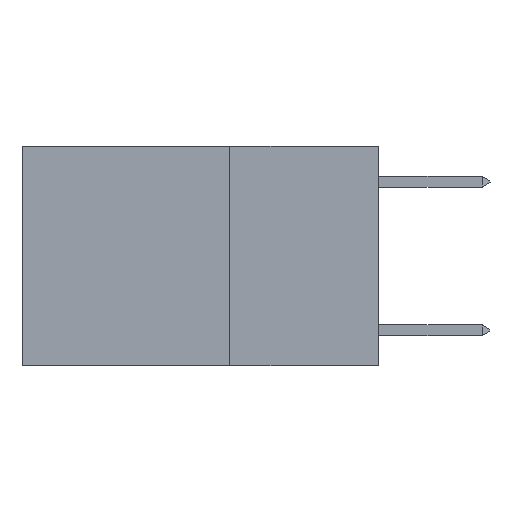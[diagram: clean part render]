
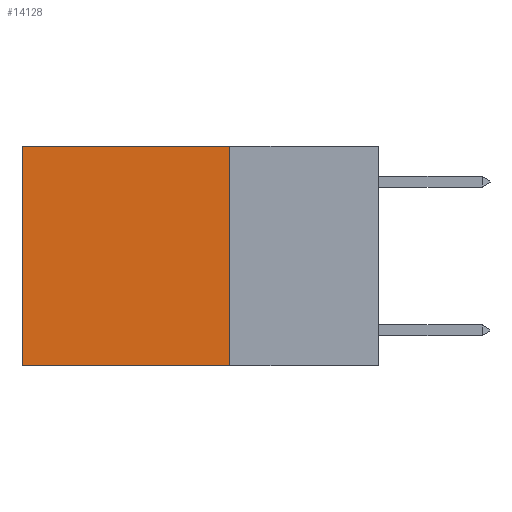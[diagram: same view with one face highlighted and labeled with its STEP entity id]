
A CAD part, left-side view. The second image highlights one B-rep face of the part: STEP entity #14128.
In plain terms, the highlighted planar face has unit normal (-1, 0, 0).
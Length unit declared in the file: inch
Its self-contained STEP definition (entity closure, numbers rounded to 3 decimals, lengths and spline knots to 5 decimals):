
#1373 = EDGE_CURVE ( 'NONE', #7896, #14406, #5699, .T. ) ;
#2200 = ORIENTED_EDGE ( 'NONE', *, *, #1373, .T. ) ;
#2500 = PLANE ( 'NONE',  #10295 ) ;
#2777 = EDGE_CURVE ( 'NONE', #14406, #12462, #14905, .T. ) ;
#3113 = LINE ( 'NONE', #14307, #6785 ) ;
#3574 = ORIENTED_EDGE ( 'NONE', *, *, #3704, .F. ) ;
#3704 = EDGE_CURVE ( 'NONE', #7896, #12253, #3113, .T. ) ;
#3740 = DIRECTION ( 'NONE',  ( 1., 0., 0. ) ) ;
#3807 = CARTESIAN_POINT ( 'NONE',  ( 0.2625, 0.25, 0. ) ) ;
#4279 = CARTESIAN_POINT ( 'NONE',  ( 0.2625, 0.6, 0. ) ) ;
#5164 = ORIENTED_EDGE ( 'NONE', *, *, #13948, .F. ) ;
#5699 = LINE ( 'NONE', #7059, #8932 ) ;
#5845 = VECTOR ( 'NONE', #6746, 39.37008 ) ;
#6357 = CARTESIAN_POINT ( 'NONE',  ( 0.2625, 0.25, -0.37 ) ) ;
#6698 = CARTESIAN_POINT ( 'NONE',  ( 0.2625, 0.6, 0. ) ) ;
#6746 = DIRECTION ( 'NONE',  ( 0., 0., -1. ) ) ;
#6785 = VECTOR ( 'NONE', #7250, 39.37008 ) ;
#7022 = VECTOR ( 'NONE', #9453, 39.37008 ) ;
#7059 = CARTESIAN_POINT ( 'NONE',  ( 0.2625, 0.25, 0. ) ) ;
#7250 = DIRECTION ( 'NONE',  ( 0., 0., -1. ) ) ;
#7896 = VERTEX_POINT ( 'NONE', #3807 ) ;
#7949 = FACE_OUTER_BOUND ( 'NONE', #11329, .T. ) ;
#8238 = CARTESIAN_POINT ( 'NONE',  ( 0.2625, 0.25, -0.37 ) ) ;
#8932 = VECTOR ( 'NONE', #15290, 39.37008 ) ;
#9453 = DIRECTION ( 'NONE',  ( 0., 1., 0. ) ) ;
#10246 = CARTESIAN_POINT ( 'NONE',  ( 0.2625, 0.6, -0.37 ) ) ;
#10295 = AXIS2_PLACEMENT_3D ( 'NONE', #14440, #3740, #12163 ) ;
#11329 = EDGE_LOOP ( 'NONE', ( #15172, #5164, #3574, #2200 ) ) ;
#12163 = DIRECTION ( 'NONE',  ( 0., 0., -1. ) ) ;
#12253 = VERTEX_POINT ( 'NONE', #6357 ) ;
#12462 = VERTEX_POINT ( 'NONE', #10246 ) ;
#13310 = LINE ( 'NONE', #8238, #7022 ) ;
#13948 = EDGE_CURVE ( 'NONE', #12253, #12462, #13310, .T. ) ;
#14128 = ADVANCED_FACE ( 'NONE', ( #7949 ), #2500, .F. ) ;
#14307 = CARTESIAN_POINT ( 'NONE',  ( 0.2625, 0.25, 0. ) ) ;
#14406 = VERTEX_POINT ( 'NONE', #6698 ) ;
#14440 = CARTESIAN_POINT ( 'NONE',  ( 0.2625, 0.25, 0. ) ) ;
#14905 = LINE ( 'NONE', #4279, #5845 ) ;
#15172 = ORIENTED_EDGE ( 'NONE', *, *, #2777, .T. ) ;
#15290 = DIRECTION ( 'NONE',  ( 0., 1., 0. ) ) ;
